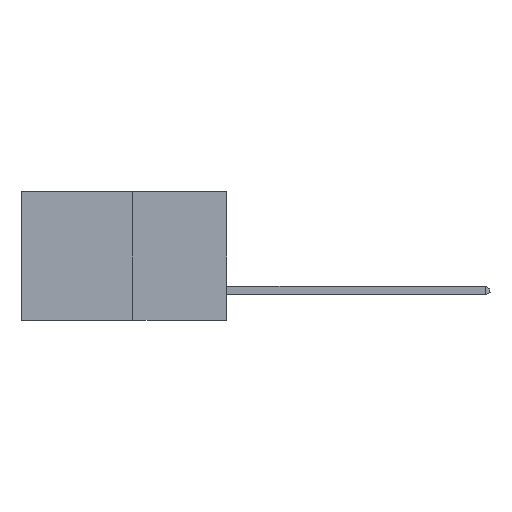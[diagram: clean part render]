
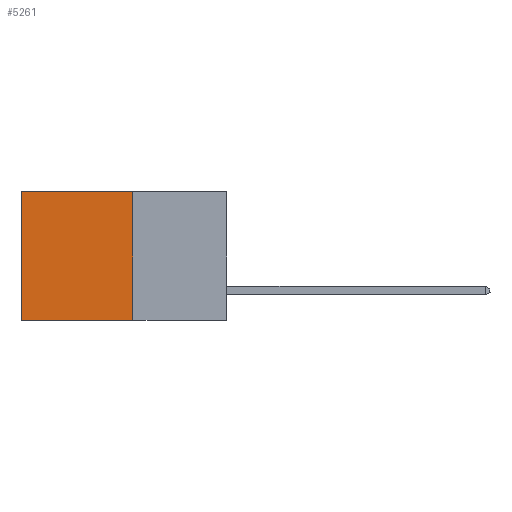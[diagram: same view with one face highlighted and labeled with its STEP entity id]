
A CAD part, left-side view. The second image highlights one B-rep face of the part: STEP entity #5261.
In plain terms, the highlighted planar face has unit normal (-1, 0, 0).
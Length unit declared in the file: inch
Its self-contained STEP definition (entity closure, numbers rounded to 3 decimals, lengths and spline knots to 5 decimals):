
#1234 = CARTESIAN_POINT ( 'NONE',  ( 0.277, 0.59, 0. ) ) ;
#2430 = ORIENTED_EDGE ( 'NONE', *, *, #12234, .F. ) ;
#2932 = DIRECTION ( 'NONE',  ( 0., 1., 0. ) ) ;
#3249 = LINE ( 'NONE', #17469, #20129 ) ;
#3800 = EDGE_CURVE ( 'NONE', #20530, #14453, #13400, .T. ) ;
#3874 = EDGE_LOOP ( 'NONE', ( #18037, #10391, #2430, #10774 ) ) ;
#4257 = LINE ( 'NONE', #9610, #8249 ) ;
#5261 = ADVANCED_FACE ( 'NONE', ( #15090 ), #17557, .F. ) ;
#6036 = DIRECTION ( 'NONE',  ( 0., 1., 0. ) ) ;
#6295 = DIRECTION ( 'NONE',  ( 0., 0., -1. ) ) ;
#7826 = EDGE_CURVE ( 'NONE', #16420, #20530, #9704, .T. ) ;
#8249 = VECTOR ( 'NONE', #6295, 39.37008 ) ;
#9203 = VECTOR ( 'NONE', #2932, 39.37008 ) ;
#9610 = CARTESIAN_POINT ( 'NONE',  ( 0.277, 0.27, -0.37 ) ) ;
#9704 = LINE ( 'NONE', #11355, #9203 ) ;
#9752 = CARTESIAN_POINT ( 'NONE',  ( 0.277, 0.27, -0.37 ) ) ;
#10375 = VERTEX_POINT ( 'NONE', #9752 ) ;
#10391 = ORIENTED_EDGE ( 'NONE', *, *, #11432, .F. ) ;
#10511 = DIRECTION ( 'NONE',  ( 0., 0., -1. ) ) ;
#10774 = ORIENTED_EDGE ( 'NONE', *, *, #7826, .T. ) ;
#11355 = CARTESIAN_POINT ( 'NONE',  ( 0.277, 0.27, 0. ) ) ;
#11432 = EDGE_CURVE ( 'NONE', #10375, #14453, #3249, .T. ) ;
#12234 = EDGE_CURVE ( 'NONE', #16420, #10375, #4257, .T. ) ;
#13341 = CARTESIAN_POINT ( 'NONE',  ( 0.277, 0.59, -0.37 ) ) ;
#13400 = LINE ( 'NONE', #13341, #17672 ) ;
#14341 = CARTESIAN_POINT ( 'NONE',  ( 0.277, 0.59, -0.37 ) ) ;
#14453 = VERTEX_POINT ( 'NONE', #14341 ) ;
#15007 = AXIS2_PLACEMENT_3D ( 'NONE', #17534, #17489, #17484 ) ;
#15090 = FACE_OUTER_BOUND ( 'NONE', #3874, .T. ) ;
#16420 = VERTEX_POINT ( 'NONE', #19271 ) ;
#17469 = CARTESIAN_POINT ( 'NONE',  ( 0.277, 0.27, -0.37 ) ) ;
#17484 = DIRECTION ( 'NONE',  ( 0., 0., -1. ) ) ;
#17489 = DIRECTION ( 'NONE',  ( 1., 0., 0. ) ) ;
#17534 = CARTESIAN_POINT ( 'NONE',  ( 0.277, 0.27, -0.37 ) ) ;
#17557 = PLANE ( 'NONE',  #15007 ) ;
#17672 = VECTOR ( 'NONE', #10511, 39.37008 ) ;
#18037 = ORIENTED_EDGE ( 'NONE', *, *, #3800, .T. ) ;
#19271 = CARTESIAN_POINT ( 'NONE',  ( 0.277, 0.27, 0. ) ) ;
#20129 = VECTOR ( 'NONE', #6036, 39.37008 ) ;
#20530 = VERTEX_POINT ( 'NONE', #1234 ) ;
